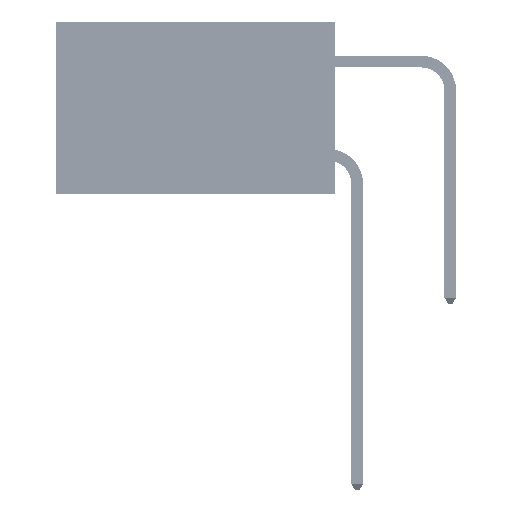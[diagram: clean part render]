
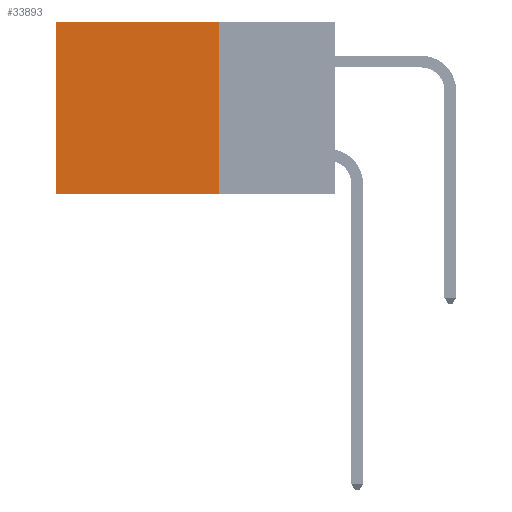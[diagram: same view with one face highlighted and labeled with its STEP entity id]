
A CAD part, left-side view. The second image highlights one B-rep face of the part: STEP entity #33893.
In plain terms, the highlighted planar face has unit normal (-1, 0, 0).
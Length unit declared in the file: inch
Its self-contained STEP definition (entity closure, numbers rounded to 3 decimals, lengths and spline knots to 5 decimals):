
#492 = CARTESIAN_POINT ( 'NONE',  ( 0.2875, 0.6, 0. ) ) ;
#1936 = CARTESIAN_POINT ( 'NONE',  ( 0.2875, 0.25, 0. ) ) ;
#2366 = VECTOR ( 'NONE', #16722, 39.37008 ) ;
#4900 = EDGE_CURVE ( 'NONE', #13987, #41570, #44197, .T. ) ;
#9055 = CARTESIAN_POINT ( 'NONE',  ( 0.2875, 0.25, -0.37 ) ) ;
#13807 = EDGE_LOOP ( 'NONE', ( #33902, #25481, #35393, #23155 ) ) ;
#13987 = VERTEX_POINT ( 'NONE', #48976 ) ;
#15327 = LINE ( 'NONE', #50192, #28655 ) ;
#16722 = DIRECTION ( 'NONE',  ( 0., 0., -1. ) ) ;
#17332 = PLANE ( 'NONE',  #32773 ) ;
#17848 = VERTEX_POINT ( 'NONE', #42397 ) ;
#20736 = VECTOR ( 'NONE', #24702, 39.37008 ) ;
#23155 = ORIENTED_EDGE ( 'NONE', *, *, #28932, .T. ) ;
#23698 = LINE ( 'NONE', #32127, #2366 ) ;
#24702 = DIRECTION ( 'NONE',  ( 0., 1., 0. ) ) ;
#25481 = ORIENTED_EDGE ( 'NONE', *, *, #4900, .F. ) ;
#25544 = DIRECTION ( 'NONE',  ( 1., 0., 0. ) ) ;
#28655 = VECTOR ( 'NONE', #43276, 39.37008 ) ;
#28932 = EDGE_CURVE ( 'NONE', #17848, #30192, #48884, .T. ) ;
#29873 = DIRECTION ( 'NONE',  ( 0., 1., 0. ) ) ;
#30192 = VERTEX_POINT ( 'NONE', #492 ) ;
#32127 = CARTESIAN_POINT ( 'NONE',  ( 0.2875, 0.6, 0. ) ) ;
#32773 = AXIS2_PLACEMENT_3D ( 'NONE', #1936, #25544, #41179 ) ;
#33483 = CARTESIAN_POINT ( 'NONE',  ( 0.2875, 0.25, 0. ) ) ;
#33515 = EDGE_CURVE ( 'NONE', #17848, #13987, #15327, .T. ) ;
#33893 = ADVANCED_FACE ( 'NONE', ( #45269 ), #17332, .F. ) ;
#33902 = ORIENTED_EDGE ( 'NONE', *, *, #49471, .T. ) ;
#34640 = CARTESIAN_POINT ( 'NONE',  ( 0.2875, 0.6, -0.37 ) ) ;
#35393 = ORIENTED_EDGE ( 'NONE', *, *, #33515, .F. ) ;
#38924 = VECTOR ( 'NONE', #29873, 39.37008 ) ;
#41179 = DIRECTION ( 'NONE',  ( 0., 0., -1. ) ) ;
#41570 = VERTEX_POINT ( 'NONE', #34640 ) ;
#42397 = CARTESIAN_POINT ( 'NONE',  ( 0.2875, 0.25, 0. ) ) ;
#43276 = DIRECTION ( 'NONE',  ( 0., 0., -1. ) ) ;
#44197 = LINE ( 'NONE', #9055, #20736 ) ;
#45269 = FACE_OUTER_BOUND ( 'NONE', #13807, .T. ) ;
#48884 = LINE ( 'NONE', #33483, #38924 ) ;
#48976 = CARTESIAN_POINT ( 'NONE',  ( 0.2875, 0.25, -0.37 ) ) ;
#49471 = EDGE_CURVE ( 'NONE', #30192, #41570, #23698, .T. ) ;
#50192 = CARTESIAN_POINT ( 'NONE',  ( 0.2875, 0.25, 0. ) ) ;
